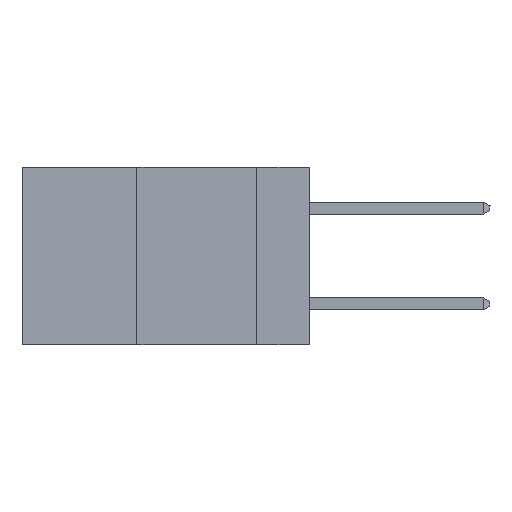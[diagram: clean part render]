
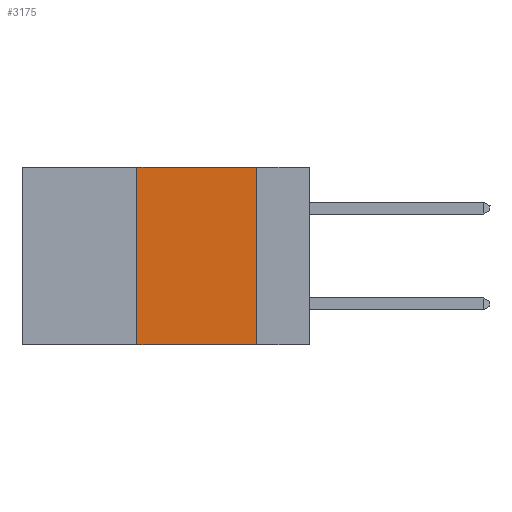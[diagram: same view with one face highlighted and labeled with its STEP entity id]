
A CAD part, left-side view. The second image highlights one B-rep face of the part: STEP entity #3175.
In plain terms, the highlighted planar face has unit normal (-1, 0, 0).
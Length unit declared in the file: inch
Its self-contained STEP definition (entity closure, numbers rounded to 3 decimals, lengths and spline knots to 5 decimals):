
#1004 = CARTESIAN_POINT ( 'NONE',  ( 0., 0.6, -0.37 ) ) ;
#1379 = EDGE_CURVE ( 'NONE', #7636, #9634, #5576, .T. ) ;
#2043 = VECTOR ( 'NONE', #4035, 39.37008 ) ;
#2336 = ORIENTED_EDGE ( 'NONE', *, *, #1379, .F. ) ;
#3175 = ADVANCED_FACE ( 'NONE', ( #16477 ), #4414, .F. ) ;
#3486 = EDGE_LOOP ( 'NONE', ( #2336, #15409, #8679, #15809 ) ) ;
#4035 = DIRECTION ( 'NONE',  ( 0., -1., 0. ) ) ;
#4414 = PLANE ( 'NONE',  #4777 ) ;
#4777 = AXIS2_PLACEMENT_3D ( 'NONE', #15602, #17020, #15668 ) ;
#5576 = LINE ( 'NONE', #6745, #5998 ) ;
#5773 = DIRECTION ( 'NONE',  ( 0., 0., 1. ) ) ;
#5998 = VECTOR ( 'NONE', #11564, 39.37008 ) ;
#6339 = EDGE_CURVE ( 'NONE', #16430, #7636, #17403, .T. ) ;
#6745 = CARTESIAN_POINT ( 'NONE',  ( 0., 0.11, 0. ) ) ;
#7636 = VERTEX_POINT ( 'NONE', #12128 ) ;
#7963 = CARTESIAN_POINT ( 'NONE',  ( 0., 0.11, -0.37 ) ) ;
#8624 = VECTOR ( 'NONE', #17994, 39.37008 ) ;
#8679 = ORIENTED_EDGE ( 'NONE', *, *, #8718, .F. ) ;
#8718 = EDGE_CURVE ( 'NONE', #11382, #16430, #12753, .T. ) ;
#9634 = VERTEX_POINT ( 'NONE', #7963 ) ;
#11382 = VERTEX_POINT ( 'NONE', #16139 ) ;
#11564 = DIRECTION ( 'NONE',  ( 0., 0., -1. ) ) ;
#12128 = CARTESIAN_POINT ( 'NONE',  ( 0., 0.11, 0. ) ) ;
#12753 = LINE ( 'NONE', #13921, #16475 ) ;
#12978 = CARTESIAN_POINT ( 'NONE',  ( 0., 0.36, 0. ) ) ;
#13921 = CARTESIAN_POINT ( 'NONE',  ( 0., 0.36, 0. ) ) ;
#15108 = LINE ( 'NONE', #1004, #8624 ) ;
#15409 = ORIENTED_EDGE ( 'NONE', *, *, #6339, .F. ) ;
#15602 = CARTESIAN_POINT ( 'NONE',  ( 0., 0.6, 0. ) ) ;
#15668 = DIRECTION ( 'NONE',  ( 0., 0., -1. ) ) ;
#15809 = ORIENTED_EDGE ( 'NONE', *, *, #17834, .T. ) ;
#16139 = CARTESIAN_POINT ( 'NONE',  ( 0., 0.36, -0.37 ) ) ;
#16383 = CARTESIAN_POINT ( 'NONE',  ( 0., 0.6, 0. ) ) ;
#16430 = VERTEX_POINT ( 'NONE', #12978 ) ;
#16475 = VECTOR ( 'NONE', #5773, 39.37008 ) ;
#16477 = FACE_OUTER_BOUND ( 'NONE', #3486, .T. ) ;
#17020 = DIRECTION ( 'NONE',  ( 1., 0., 0. ) ) ;
#17403 = LINE ( 'NONE', #16383, #2043 ) ;
#17834 = EDGE_CURVE ( 'NONE', #11382, #9634, #15108, .T. ) ;
#17994 = DIRECTION ( 'NONE',  ( 0., -1., 0. ) ) ;
